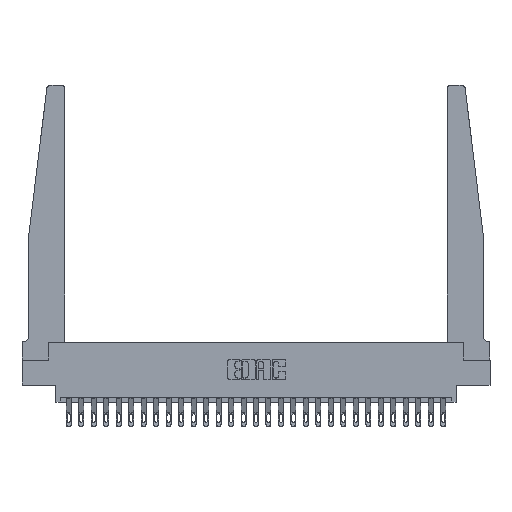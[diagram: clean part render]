
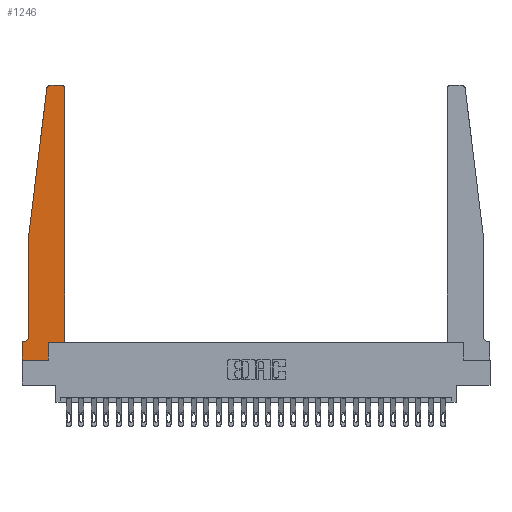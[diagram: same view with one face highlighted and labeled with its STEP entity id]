
A CAD part, top view. The second image highlights one B-rep face of the part: STEP entity #1246.
In plain terms, the highlighted planar face has unit normal (0, 0, 1).
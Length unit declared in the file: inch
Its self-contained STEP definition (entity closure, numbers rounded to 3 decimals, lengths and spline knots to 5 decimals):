
#188 = DIRECTION ( 'NONE',  ( 0., -1., 0. ) ) ;
#315 = CARTESIAN_POINT ( 'NONE',  ( 0.395, 2.75, 0.37 ) ) ;
#1036 = AXIS2_PLACEMENT_3D ( 'NONE', #5268, #20104, #3610 ) ;
#1108 = PLANE ( 'NONE',  #1036 ) ;
#1246 = ADVANCED_FACE ( 'NONE', ( #12063 ), #1108, .T. ) ;
#1404 = ORIENTED_EDGE ( 'NONE', *, *, #25983, .T. ) ;
#1814 = ORIENTED_EDGE ( 'NONE', *, *, #13315, .T. ) ;
#1864 = DIRECTION ( 'NONE',  ( 1., 0., 0. ) ) ;
#2229 = EDGE_CURVE ( 'NONE', #6084, #7468, #7726, .T. ) ;
#2281 = VERTEX_POINT ( 'NONE', #8367 ) ;
#2520 = DIRECTION ( 'NONE',  ( 0., 1., 0. ) ) ;
#2592 = DIRECTION ( 'NONE',  ( 0., -1., 0. ) ) ;
#2995 = VERTEX_POINT ( 'NONE', #5006 ) ;
#3227 = EDGE_CURVE ( 'NONE', #8704, #20499, #12442, .T. ) ;
#3263 = EDGE_CURVE ( 'NONE', #7468, #22525, #11328, .T. ) ;
#3610 = DIRECTION ( 'NONE',  ( 1., 0., 0. ) ) ;
#4037 = ORIENTED_EDGE ( 'NONE', *, *, #7332, .T. ) ;
#4191 = EDGE_CURVE ( 'NONE', #12710, #5378, #17215, .T. ) ;
#4726 = CARTESIAN_POINT ( 'NONE',  ( 0.24675, 2.72367, 0.37 ) ) ;
#5006 = CARTESIAN_POINT ( 'NONE',  ( 0.065, 0.2375, 0.37 ) ) ;
#5039 = DIRECTION ( 'NONE',  ( 1., 0., 0. ) ) ;
#5210 = AXIS2_PLACEMENT_3D ( 'NONE', #25538, #16791, #12654 ) ;
#5268 = CARTESIAN_POINT ( 'NONE',  ( 0., 0.1875, 0.37 ) ) ;
#5315 = DIRECTION ( 'NONE',  ( 0., 0., -1. ) ) ;
#5378 = VERTEX_POINT ( 'NONE', #26049 ) ;
#5512 = CARTESIAN_POINT ( 'NONE',  ( 0.2605, 0.18, 0.37 ) ) ;
#6036 = DIRECTION ( 'NONE',  ( -0.122, -0.992, 0. ) ) ;
#6084 = VERTEX_POINT ( 'NONE', #20322 ) ;
#6154 = EDGE_LOOP ( 'NONE', ( #24956, #13642, #1404, #20725, #22059, #9652, #8638, #10303, #4037, #9378, #1814, #21368 ) ) ;
#6974 = CARTESIAN_POINT ( 'NONE',  ( 0.425, 0.18, 0.37 ) ) ;
#7259 = CARTESIAN_POINT ( 'NONE',  ( 0.015, 0.2375, 0.37 ) ) ;
#7332 = EDGE_CURVE ( 'NONE', #5378, #8508, #26093, .T. ) ;
#7468 = VERTEX_POINT ( 'NONE', #315 ) ;
#7726 = CIRCLE ( 'NONE', #9930, 0.03 ) ;
#8367 = CARTESIAN_POINT ( 'NONE',  ( 0.065, 1.25, 0.37 ) ) ;
#8398 = CARTESIAN_POINT ( 'NONE',  ( 0.065, 0.1875, 0.37 ) ) ;
#8508 = VERTEX_POINT ( 'NONE', #5512 ) ;
#8638 = ORIENTED_EDGE ( 'NONE', *, *, #12831, .T. ) ;
#8704 = VERTEX_POINT ( 'NONE', #16593 ) ;
#9028 = LINE ( 'NONE', #11521, #10118 ) ;
#9378 = ORIENTED_EDGE ( 'NONE', *, *, #11598, .T. ) ;
#9652 = ORIENTED_EDGE ( 'NONE', *, *, #3227, .T. ) ;
#9930 = AXIS2_PLACEMENT_3D ( 'NONE', #22675, #24736, #1864 ) ;
#10118 = VECTOR ( 'NONE', #2520, 39.37008 ) ;
#10303 = ORIENTED_EDGE ( 'NONE', *, *, #4191, .T. ) ;
#11328 = LINE ( 'NONE', #19776, #17773 ) ;
#11521 = CARTESIAN_POINT ( 'NONE',  ( 0.425, 0.18, 0.37 ) ) ;
#11598 = EDGE_CURVE ( 'NONE', #8508, #16367, #15296, .T. ) ;
#12063 = FACE_OUTER_BOUND ( 'NONE', #6154, .T. ) ;
#12442 = LINE ( 'NONE', #8398, #20447 ) ;
#12654 = DIRECTION ( 'NONE',  ( 1., 0., 0. ) ) ;
#12710 = VERTEX_POINT ( 'NONE', #26540 ) ;
#12718 = DIRECTION ( 'NONE',  ( -1., 0., 0. ) ) ;
#12786 = DIRECTION ( 'NONE',  ( 1., 0., 0. ) ) ;
#12831 = EDGE_CURVE ( 'NONE', #20499, #12710, #17239, .T. ) ;
#12952 = CARTESIAN_POINT ( 'NONE',  ( 0., 0., 0.37 ) ) ;
#13161 = EDGE_CURVE ( 'NONE', #22525, #26383, #18498, .T. ) ;
#13315 = EDGE_CURVE ( 'NONE', #16367, #6084, #9028, .T. ) ;
#13427 = VECTOR ( 'NONE', #5039, 39.37008 ) ;
#13482 = VECTOR ( 'NONE', #6036, 39.37008 ) ;
#13642 = ORIENTED_EDGE ( 'NONE', *, *, #13161, .T. ) ;
#15296 = LINE ( 'NONE', #6974, #13427 ) ;
#15604 = CARTESIAN_POINT ( 'NONE',  ( 0.065, 1.25, 0.37 ) ) ;
#16349 = EDGE_CURVE ( 'NONE', #2281, #2995, #26147, .T. ) ;
#16367 = VERTEX_POINT ( 'NONE', #22009 ) ;
#16398 = VECTOR ( 'NONE', #188, 39.37008 ) ;
#16593 = CARTESIAN_POINT ( 'NONE',  ( 0.015, 0.1875, 0.37 ) ) ;
#16791 = DIRECTION ( 'NONE',  ( 0., 0., 1. ) ) ;
#17215 = LINE ( 'NONE', #25803, #18145 ) ;
#17239 = LINE ( 'NONE', #12952, #16398 ) ;
#17682 = DIRECTION ( 'NONE',  ( -1., 0., 0. ) ) ;
#17773 = VECTOR ( 'NONE', #17682, 39.37008 ) ;
#17779 = DIRECTION ( 'NONE',  ( 0., 1., 0. ) ) ;
#17802 = DIRECTION ( 'NONE',  ( -1., 0., 0. ) ) ;
#18145 = VECTOR ( 'NONE', #12786, 39.37008 ) ;
#18190 = VECTOR ( 'NONE', #2592, 39.37008 ) ;
#18498 = CIRCLE ( 'NONE', #5210, 0.03 ) ;
#19585 = CARTESIAN_POINT ( 'NONE',  ( 0.2605, 0.18, 0.37 ) ) ;
#19776 = CARTESIAN_POINT ( 'NONE',  ( 0.25, 2.75, 0.37 ) ) ;
#20104 = DIRECTION ( 'NONE',  ( 0., 0., 1. ) ) ;
#20322 = CARTESIAN_POINT ( 'NONE',  ( 0.425, 2.72, 0.37 ) ) ;
#20447 = VECTOR ( 'NONE', #12718, 39.37008 ) ;
#20499 = VERTEX_POINT ( 'NONE', #23112 ) ;
#20725 = ORIENTED_EDGE ( 'NONE', *, *, #16349, .T. ) ;
#21368 = ORIENTED_EDGE ( 'NONE', *, *, #2229, .T. ) ;
#21384 = AXIS2_PLACEMENT_3D ( 'NONE', #7259, #5315, #17802 ) ;
#22009 = CARTESIAN_POINT ( 'NONE',  ( 0.425, 0.18, 0.37 ) ) ;
#22059 = ORIENTED_EDGE ( 'NONE', *, *, #22414, .T. ) ;
#22342 = VECTOR ( 'NONE', #17779, 39.37008 ) ;
#22392 = CARTESIAN_POINT ( 'NONE',  ( 0.27653, 2.75, 0.37 ) ) ;
#22414 = EDGE_CURVE ( 'NONE', #2995, #8704, #26687, .T. ) ;
#22525 = VERTEX_POINT ( 'NONE', #22392 ) ;
#22675 = CARTESIAN_POINT ( 'NONE',  ( 0.395, 2.72, 0.37 ) ) ;
#23112 = CARTESIAN_POINT ( 'NONE',  ( 0., 0.1875, 0.37 ) ) ;
#23754 = CARTESIAN_POINT ( 'NONE',  ( 0.065, 1.25, 0.37 ) ) ;
#24736 = DIRECTION ( 'NONE',  ( 0., 0., 1. ) ) ;
#24956 = ORIENTED_EDGE ( 'NONE', *, *, #3263, .T. ) ;
#25033 = LINE ( 'NONE', #23754, #13482 ) ;
#25538 = CARTESIAN_POINT ( 'NONE',  ( 0.27653, 2.72, 0.37 ) ) ;
#25803 = CARTESIAN_POINT ( 'NONE',  ( 0., 0., 0.37 ) ) ;
#25983 = EDGE_CURVE ( 'NONE', #26383, #2281, #25033, .T. ) ;
#26049 = CARTESIAN_POINT ( 'NONE',  ( 0.2605, 0., 0.37 ) ) ;
#26093 = LINE ( 'NONE', #19585, #22342 ) ;
#26147 = LINE ( 'NONE', #15604, #18190 ) ;
#26383 = VERTEX_POINT ( 'NONE', #4726 ) ;
#26540 = CARTESIAN_POINT ( 'NONE',  ( 0., 0., 0.37 ) ) ;
#26687 = CIRCLE ( 'NONE', #21384, 0.05 ) ;
